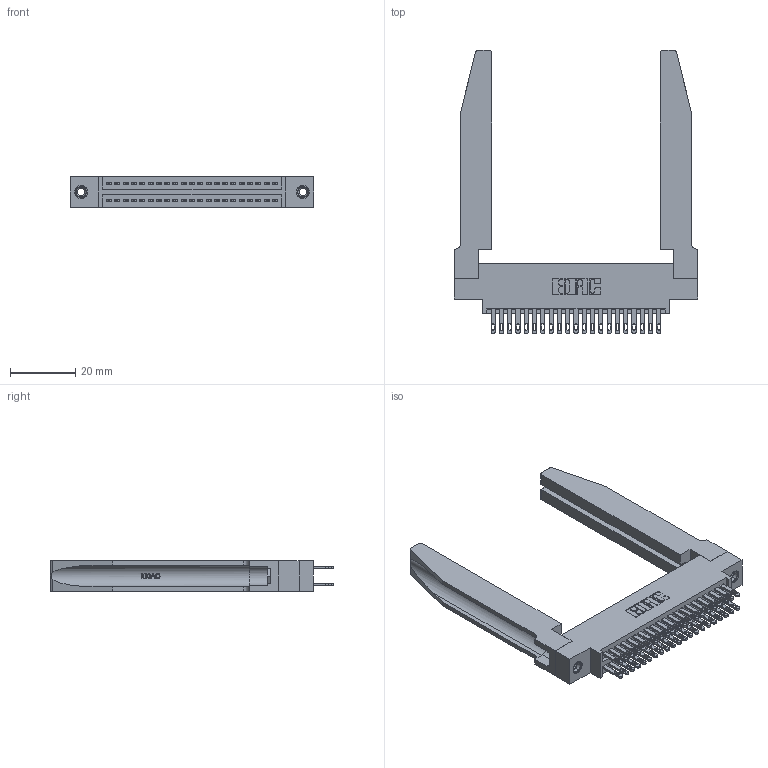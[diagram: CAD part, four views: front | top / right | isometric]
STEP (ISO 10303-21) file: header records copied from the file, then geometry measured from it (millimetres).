
FILE_DESCRIPTION (( 'STEP AP203' ), '1' );
FILE_NAME ('345-042-500-878.STEP', '2019-10-28T19:09:33', ( '' ), ( '' ), 'SwSTEP 2.0', 'SolidWorks 2016', '' );
FILE_SCHEMA (( 'CONFIG_CONTROL_DESIGN' ));
Length unit declared in the file: inch
Products named in the file (5): 345-292-001_345-293-100; 345 Part_0.170 Offset - 0.156 Dia-TH; 345-220-078_345-220-078; 345-250-001_345-250-001-102; 345-042-500-878
Assembly tree (47 placements, depth 2):
  345-042-500-878
    345 Part_0.170 Offset - 0.156 Dia-TH
    345-292-001_345-293-100  x42
    345-250-001_345-250-001-102  x2
    345-220-078_345-220-078  x2
Bounding box: 74.57 x 86.79 x 9.4 mm (x, y, z)
Volume: 14834.7 mm3; surface area: 17445.7 mm2
Topology: 47 solids, 47 shells, 2296 faces, 6883 edges, 4578 vertices
Faces by surface type: plane 1360, cylinder 884, bspline 36, cone 12, torus 4
Entity records: 24106 total; most frequent: CARTESIAN_POINT 4979, ORIENTED_EDGE 3810, DIRECTION 3411, EDGE_CURVE 1905, LINE 1591, VECTOR 1591, VERTEX_POINT 1264, AXIS2_PLACEMENT_3D 910
